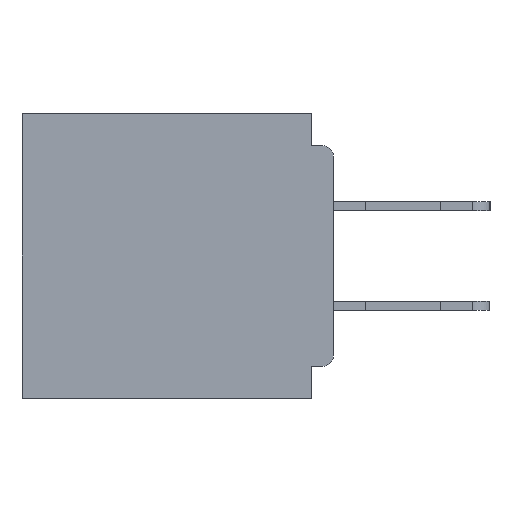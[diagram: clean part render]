
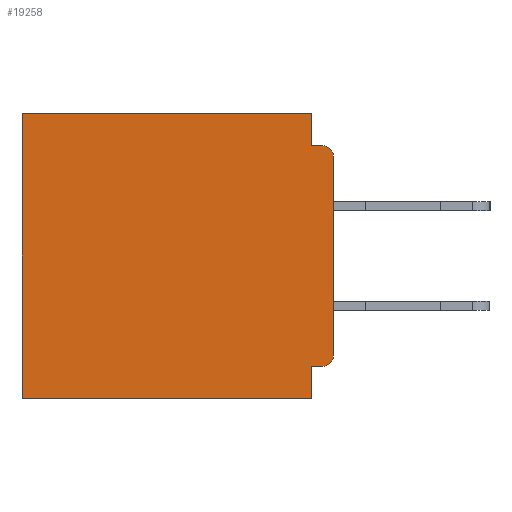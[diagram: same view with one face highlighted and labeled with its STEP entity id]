
A CAD part, left-side view. The second image highlights one B-rep face of the part: STEP entity #19258.
In plain terms, the highlighted planar face has unit normal (-1, 0, 0).
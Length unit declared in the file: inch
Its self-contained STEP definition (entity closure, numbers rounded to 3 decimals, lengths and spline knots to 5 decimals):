
#508 = CIRCLE ( 'NONE', #15704, 0.015 ) ;
#801 = DIRECTION ( 'NONE',  ( 0., 1., 0. ) ) ;
#2013 = EDGE_CURVE ( 'NONE', #33886, #28750, #26164, .T. ) ;
#2074 = ORIENTED_EDGE ( 'NONE', *, *, #33208, .F. ) ;
#2443 = VERTEX_POINT ( 'NONE', #19915 ) ;
#2781 = CIRCLE ( 'NONE', #22994, 0.015 ) ;
#3109 = VECTOR ( 'NONE', #801, 39.37008 ) ;
#4114 = CARTESIAN_POINT ( 'NONE',  ( 0.3, 0.437, -0.4 ) ) ;
#4762 = CARTESIAN_POINT ( 'NONE',  ( 0.3, 0., -0.045 ) ) ;
#5427 = DIRECTION ( 'NONE',  ( 0., 1., 0. ) ) ;
#6825 = VERTEX_POINT ( 'NONE', #20699 ) ;
#7102 = VECTOR ( 'NONE', #35158, 39.37008 ) ;
#7866 = VERTEX_POINT ( 'NONE', #19829 ) ;
#8000 = LINE ( 'NONE', #43052, #27019 ) ;
#8050 = EDGE_CURVE ( 'NONE', #28750, #7866, #35624, .T. ) ;
#8346 = DIRECTION ( 'NONE',  ( -1., 0., 0. ) ) ;
#8701 = ORIENTED_EDGE ( 'NONE', *, *, #36488, .T. ) ;
#9020 = DIRECTION ( 'NONE',  ( -1., 0., 0. ) ) ;
#10153 = VERTEX_POINT ( 'NONE', #34423 ) ;
#10413 = EDGE_CURVE ( 'NONE', #43311, #10153, #8000, .T. ) ;
#10843 = LINE ( 'NONE', #4762, #30991 ) ;
#11220 = ORIENTED_EDGE ( 'NONE', *, *, #18815, .F. ) ;
#12612 = LINE ( 'NONE', #36473, #3109 ) ;
#12882 = ORIENTED_EDGE ( 'NONE', *, *, #10413, .F. ) ;
#14092 = PLANE ( 'NONE',  #43622 ) ;
#14481 = ORIENTED_EDGE ( 'NONE', *, *, #24519, .T. ) ;
#15704 = AXIS2_PLACEMENT_3D ( 'NONE', #30447, #9020, #34007 ) ;
#15949 = CARTESIAN_POINT ( 'NONE',  ( 0.3, 0., -0.06 ) ) ;
#16364 = ORIENTED_EDGE ( 'NONE', *, *, #8050, .F. ) ;
#16578 = VECTOR ( 'NONE', #21712, 39.37008 ) ;
#17204 = ORIENTED_EDGE ( 'NONE', *, *, #31982, .F. ) ;
#17674 = DIRECTION ( 'NONE',  ( 0., 0., -1. ) ) ;
#18275 = LINE ( 'NONE', #26964, #36172 ) ;
#18815 = EDGE_CURVE ( 'NONE', #10153, #6825, #10843, .T. ) ;
#19258 = ADVANCED_FACE ( 'NONE', ( #20286 ), #14092, .F. ) ;
#19829 = CARTESIAN_POINT ( 'NONE',  ( 0.3, 0.031, -0.4 ) ) ;
#19915 = CARTESIAN_POINT ( 'NONE',  ( 0.3, 0., -0.34 ) ) ;
#20108 = CARTESIAN_POINT ( 'NONE',  ( 0.3, 0.015, -0.355 ) ) ;
#20286 = FACE_OUTER_BOUND ( 'NONE', #35166, .T. ) ;
#20699 = CARTESIAN_POINT ( 'NONE',  ( 0.3, 0.015, -0.045 ) ) ;
#21336 = VECTOR ( 'NONE', #40193, 39.37008 ) ;
#21712 = DIRECTION ( 'NONE',  ( 0., 1., 0. ) ) ;
#21754 = DIRECTION ( 'NONE',  ( 0., 0., -1. ) ) ;
#22253 = CARTESIAN_POINT ( 'NONE',  ( 0.3, 0.031, -0.355 ) ) ;
#22868 = CARTESIAN_POINT ( 'NONE',  ( 0.3, 0.437, 0. ) ) ;
#22994 = AXIS2_PLACEMENT_3D ( 'NONE', #29791, #8346, #33329 ) ;
#23379 = ORIENTED_EDGE ( 'NONE', *, *, #35837, .T. ) ;
#23452 = VECTOR ( 'NONE', #5427, 39.37008 ) ;
#24519 = EDGE_CURVE ( 'NONE', #33886, #2443, #508, .T. ) ;
#25465 = VERTEX_POINT ( 'NONE', #4114 ) ;
#26164 = LINE ( 'NONE', #42904, #16578 ) ;
#26896 = CARTESIAN_POINT ( 'NONE',  ( 0.3, 0., -0.4 ) ) ;
#26964 = CARTESIAN_POINT ( 'NONE',  ( 0.3, 0., -0.4 ) ) ;
#27019 = VECTOR ( 'NONE', #21754, 39.37008 ) ;
#28750 = VERTEX_POINT ( 'NONE', #22253 ) ;
#29791 = CARTESIAN_POINT ( 'NONE',  ( 0.3, 0.015, -0.06 ) ) ;
#29807 = DIRECTION ( 'NONE',  ( 0., -1., 0. ) ) ;
#30447 = CARTESIAN_POINT ( 'NONE',  ( 0.3, 0.015, -0.34 ) ) ;
#30532 = DIRECTION ( 'NONE',  ( 0., 0., -1. ) ) ;
#30862 = LINE ( 'NONE', #36665, #21336 ) ;
#30991 = VECTOR ( 'NONE', #29807, 39.37008 ) ;
#31571 = CARTESIAN_POINT ( 'NONE',  ( 0.3, 0.031, -0.4 ) ) ;
#31982 = EDGE_CURVE ( 'NONE', #7866, #25465, #32942, .T. ) ;
#32942 = LINE ( 'NONE', #26896, #23452 ) ;
#33208 = EDGE_CURVE ( 'NONE', #36586, #2443, #18275, .T. ) ;
#33329 = DIRECTION ( 'NONE',  ( 0., 0., -1. ) ) ;
#33886 = VERTEX_POINT ( 'NONE', #20108 ) ;
#34007 = DIRECTION ( 'NONE',  ( 0., 0., -1. ) ) ;
#34423 = CARTESIAN_POINT ( 'NONE',  ( 0.3, 0.031, -0.045 ) ) ;
#35158 = DIRECTION ( 'NONE',  ( 0., 0., -1. ) ) ;
#35166 = EDGE_LOOP ( 'NONE', ( #2074, #8701, #11220, #12882, #45169, #23379, #17204, #16364, #43347, #14481 ) ) ;
#35624 = LINE ( 'NONE', #31571, #7102 ) ;
#35837 = EDGE_CURVE ( 'NONE', #36577, #25465, #30862, .T. ) ;
#36172 = VECTOR ( 'NONE', #30532, 39.37008 ) ;
#36473 = CARTESIAN_POINT ( 'NONE',  ( 0.3, 0., 0. ) ) ;
#36488 = EDGE_CURVE ( 'NONE', #36586, #6825, #2781, .T. ) ;
#36577 = VERTEX_POINT ( 'NONE', #22868 ) ;
#36586 = VERTEX_POINT ( 'NONE', #15949 ) ;
#36665 = CARTESIAN_POINT ( 'NONE',  ( 0.3, 0.437, -0.4 ) ) ;
#39016 = DIRECTION ( 'NONE',  ( 1., 0., 0. ) ) ;
#39513 = EDGE_CURVE ( 'NONE', #43311, #36577, #12612, .T. ) ;
#40193 = DIRECTION ( 'NONE',  ( 0., 0., -1. ) ) ;
#42904 = CARTESIAN_POINT ( 'NONE',  ( 0.3, 0., -0.355 ) ) ;
#43052 = CARTESIAN_POINT ( 'NONE',  ( 0.3, 0.031, 0. ) ) ;
#43311 = VERTEX_POINT ( 'NONE', #44134 ) ;
#43347 = ORIENTED_EDGE ( 'NONE', *, *, #2013, .F. ) ;
#43622 = AXIS2_PLACEMENT_3D ( 'NONE', #45994, #39016, #17674 ) ;
#44134 = CARTESIAN_POINT ( 'NONE',  ( 0.3, 0.031, 0. ) ) ;
#45169 = ORIENTED_EDGE ( 'NONE', *, *, #39513, .T. ) ;
#45994 = CARTESIAN_POINT ( 'NONE',  ( 0.3, 0., -0.4 ) ) ;
